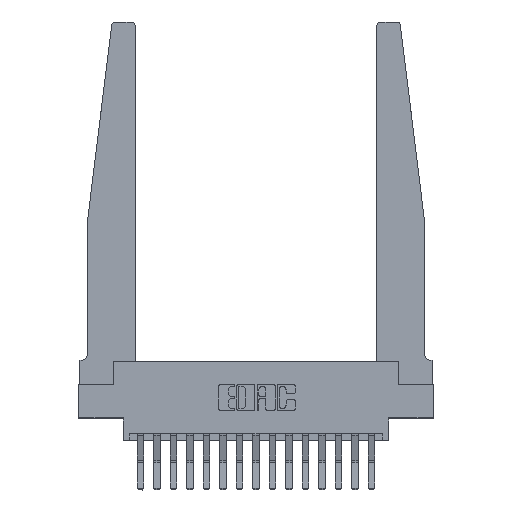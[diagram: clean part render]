
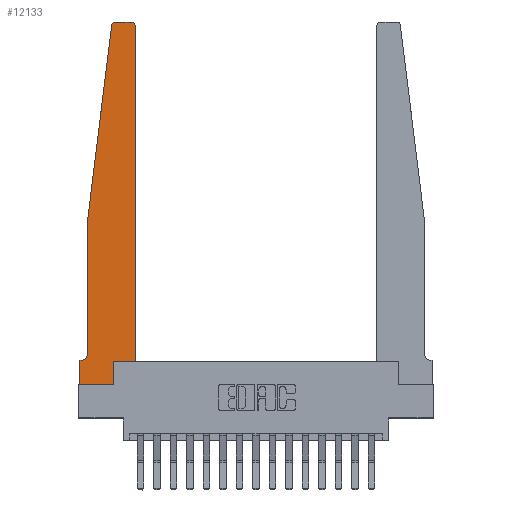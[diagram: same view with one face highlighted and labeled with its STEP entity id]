
A CAD part, top view. The second image highlights one B-rep face of the part: STEP entity #12133.
In plain terms, the highlighted planar face has unit normal (0, 0, 1).
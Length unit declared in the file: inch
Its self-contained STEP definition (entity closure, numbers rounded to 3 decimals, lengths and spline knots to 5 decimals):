
#278 = LINE ( 'NONE', #3231, #14993 ) ;
#340 = LINE ( 'NONE', #801, #17921 ) ;
#343 = EDGE_CURVE ( 'NONE', #16078, #15351, #1198, .T. ) ;
#371 = DIRECTION ( 'NONE',  ( 0., 0., 1. ) ) ;
#554 = DIRECTION ( 'NONE',  ( -0.122, -0.992, 0. ) ) ;
#667 = CARTESIAN_POINT ( 'NONE',  ( 0.25, 2.75, 0.37 ) ) ;
#709 = ORIENTED_EDGE ( 'NONE', *, *, #15627, .T. ) ;
#801 = CARTESIAN_POINT ( 'NONE',  ( 0.425, 0.18, 0.37 ) ) ;
#826 = ORIENTED_EDGE ( 'NONE', *, *, #17113, .T. ) ;
#1198 = LINE ( 'NONE', #2879, #15885 ) ;
#1217 = CIRCLE ( 'NONE', #6564, 0.03 ) ;
#1340 = VECTOR ( 'NONE', #11942, 39.37008 ) ;
#1404 = EDGE_CURVE ( 'NONE', #16367, #2263, #15848, .T. ) ;
#1773 = LINE ( 'NONE', #1954, #1340 ) ;
#1954 = CARTESIAN_POINT ( 'NONE',  ( 0., 0., 0.37 ) ) ;
#2148 = DIRECTION ( 'NONE',  ( 0., 0., -1. ) ) ;
#2263 = VERTEX_POINT ( 'NONE', #13148 ) ;
#2516 = ORIENTED_EDGE ( 'NONE', *, *, #1404, .T. ) ;
#2554 = DIRECTION ( 'NONE',  ( 0., 0., 1. ) ) ;
#2879 = CARTESIAN_POINT ( 'NONE',  ( 0.065, 1.25, 0.37 ) ) ;
#3231 = CARTESIAN_POINT ( 'NONE',  ( 0.065, 0.1875, 0.37 ) ) ;
#3321 = EDGE_CURVE ( 'NONE', #2263, #16339, #1773, .T. ) ;
#3519 = ORIENTED_EDGE ( 'NONE', *, *, #3321, .T. ) ;
#3596 = CARTESIAN_POINT ( 'NONE',  ( 0., 0., 0.37 ) ) ;
#3991 = CARTESIAN_POINT ( 'NONE',  ( 0.425, 2.72, 0.37 ) ) ;
#4060 = LINE ( 'NONE', #6442, #12583 ) ;
#4134 = DIRECTION ( 'NONE',  ( 0., -1., 0. ) ) ;
#4240 = CARTESIAN_POINT ( 'NONE',  ( 0., 0.1875, 0.37 ) ) ;
#4636 = VECTOR ( 'NONE', #10656, 39.37008 ) ;
#4926 = VECTOR ( 'NONE', #16715, 39.37008 ) ;
#5001 = DIRECTION ( 'NONE',  ( -1., 0., 0. ) ) ;
#5351 = EDGE_CURVE ( 'NONE', #16339, #17044, #12287, .T. ) ;
#5472 = VECTOR ( 'NONE', #554, 39.37008 ) ;
#6189 = CIRCLE ( 'NONE', #17028, 0.05 ) ;
#6236 = VERTEX_POINT ( 'NONE', #7649 ) ;
#6309 = CARTESIAN_POINT ( 'NONE',  ( 0.27653, 2.72, 0.37 ) ) ;
#6442 = CARTESIAN_POINT ( 'NONE',  ( 0.425, 0.18, 0.37 ) ) ;
#6564 = AXIS2_PLACEMENT_3D ( 'NONE', #6309, #16284, #7735 ) ;
#6732 = VERTEX_POINT ( 'NONE', #17470 ) ;
#7047 = EDGE_CURVE ( 'NONE', #14436, #8310, #15754, .T. ) ;
#7271 = CARTESIAN_POINT ( 'NONE',  ( 0.065, 0.2375, 0.37 ) ) ;
#7423 = CARTESIAN_POINT ( 'NONE',  ( 0.2605, 0.18, 0.37 ) ) ;
#7480 = CARTESIAN_POINT ( 'NONE',  ( 0., 0.1875, 0.37 ) ) ;
#7537 = ORIENTED_EDGE ( 'NONE', *, *, #15509, .T. ) ;
#7649 = CARTESIAN_POINT ( 'NONE',  ( 0.24675, 2.72367, 0.37 ) ) ;
#7735 = DIRECTION ( 'NONE',  ( 1., 0., 0. ) ) ;
#8127 = ORIENTED_EDGE ( 'NONE', *, *, #343, .T. ) ;
#8260 = ORIENTED_EDGE ( 'NONE', *, *, #17083, .T. ) ;
#8310 = VERTEX_POINT ( 'NONE', #12996 ) ;
#8685 = ORIENTED_EDGE ( 'NONE', *, *, #12972, .T. ) ;
#8899 = PLANE ( 'NONE',  #16308 ) ;
#8968 = ORIENTED_EDGE ( 'NONE', *, *, #16566, .T. ) ;
#9152 = ORIENTED_EDGE ( 'NONE', *, *, #7047, .T. ) ;
#9675 = CARTESIAN_POINT ( 'NONE',  ( 0.425, 0.18, 0.37 ) ) ;
#10040 = FACE_OUTER_BOUND ( 'NONE', #15019, .T. ) ;
#10363 = DIRECTION ( 'NONE',  ( 1., 0., 0. ) ) ;
#10656 = DIRECTION ( 'NONE',  ( -1., 0., 0. ) ) ;
#10708 = CARTESIAN_POINT ( 'NONE',  ( 0.015, 0.2375, 0.37 ) ) ;
#11129 = CARTESIAN_POINT ( 'NONE',  ( 0.395, 2.72, 0.37 ) ) ;
#11356 = LINE ( 'NONE', #667, #4636 ) ;
#11942 = DIRECTION ( 'NONE',  ( 1., 0., 0. ) ) ;
#12128 = DIRECTION ( 'NONE',  ( 1., 0., 0. ) ) ;
#12133 = ADVANCED_FACE ( 'NONE', ( #10040 ), #8899, .T. ) ;
#12137 = DIRECTION ( 'NONE',  ( 0., 1., 0. ) ) ;
#12149 = DIRECTION ( 'NONE',  ( -1., 0., 0. ) ) ;
#12168 = CARTESIAN_POINT ( 'NONE',  ( 0.27653, 2.75, 0.37 ) ) ;
#12287 = LINE ( 'NONE', #15037, #15589 ) ;
#12428 = ORIENTED_EDGE ( 'NONE', *, *, #14213, .T. ) ;
#12577 = DIRECTION ( 'NONE',  ( 1., 0., 0. ) ) ;
#12583 = VECTOR ( 'NONE', #12128, 39.37008 ) ;
#12972 = EDGE_CURVE ( 'NONE', #8310, #15587, #11356, .T. ) ;
#12996 = CARTESIAN_POINT ( 'NONE',  ( 0.395, 2.75, 0.37 ) ) ;
#13148 = CARTESIAN_POINT ( 'NONE',  ( 0., 0., 0.37 ) ) ;
#13339 = CARTESIAN_POINT ( 'NONE',  ( 0.065, 1.25, 0.37 ) ) ;
#13506 = CARTESIAN_POINT ( 'NONE',  ( 0.065, 1.25, 0.37 ) ) ;
#13641 = DIRECTION ( 'NONE',  ( 0., 1., 0. ) ) ;
#14213 = EDGE_CURVE ( 'NONE', #15351, #6732, #6189, .T. ) ;
#14418 = AXIS2_PLACEMENT_3D ( 'NONE', #11129, #2554, #12577 ) ;
#14436 = VERTEX_POINT ( 'NONE', #3991 ) ;
#14993 = VECTOR ( 'NONE', #5001, 39.37008 ) ;
#15019 = EDGE_LOOP ( 'NONE', ( #8685, #8968, #7537, #8127, #12428, #8260, #2516, #3519, #17203, #826, #709, #9152 ) ) ;
#15037 = CARTESIAN_POINT ( 'NONE',  ( 0.2605, 0.18, 0.37 ) ) ;
#15351 = VERTEX_POINT ( 'NONE', #7271 ) ;
#15509 = EDGE_CURVE ( 'NONE', #6236, #16078, #16390, .T. ) ;
#15587 = VERTEX_POINT ( 'NONE', #12168 ) ;
#15589 = VECTOR ( 'NONE', #12137, 39.37008 ) ;
#15627 = EDGE_CURVE ( 'NONE', #17288, #14436, #340, .T. ) ;
#15754 = CIRCLE ( 'NONE', #14418, 0.03 ) ;
#15848 = LINE ( 'NONE', #3596, #4926 ) ;
#15885 = VECTOR ( 'NONE', #4134, 39.37008 ) ;
#16078 = VERTEX_POINT ( 'NONE', #13506 ) ;
#16284 = DIRECTION ( 'NONE',  ( 0., 0., 1. ) ) ;
#16308 = AXIS2_PLACEMENT_3D ( 'NONE', #7480, #371, #10363 ) ;
#16339 = VERTEX_POINT ( 'NONE', #17014 ) ;
#16367 = VERTEX_POINT ( 'NONE', #4240 ) ;
#16390 = LINE ( 'NONE', #13339, #5472 ) ;
#16566 = EDGE_CURVE ( 'NONE', #15587, #6236, #1217, .T. ) ;
#16715 = DIRECTION ( 'NONE',  ( 0., -1., 0. ) ) ;
#17014 = CARTESIAN_POINT ( 'NONE',  ( 0.2605, 0., 0.37 ) ) ;
#17028 = AXIS2_PLACEMENT_3D ( 'NONE', #10708, #2148, #12149 ) ;
#17044 = VERTEX_POINT ( 'NONE', #7423 ) ;
#17083 = EDGE_CURVE ( 'NONE', #6732, #16367, #278, .T. ) ;
#17113 = EDGE_CURVE ( 'NONE', #17044, #17288, #4060, .T. ) ;
#17203 = ORIENTED_EDGE ( 'NONE', *, *, #5351, .T. ) ;
#17288 = VERTEX_POINT ( 'NONE', #9675 ) ;
#17470 = CARTESIAN_POINT ( 'NONE',  ( 0.015, 0.1875, 0.37 ) ) ;
#17921 = VECTOR ( 'NONE', #13641, 39.37008 ) ;
